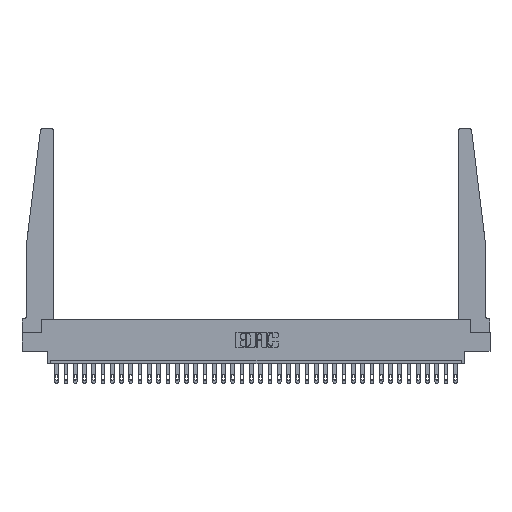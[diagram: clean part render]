
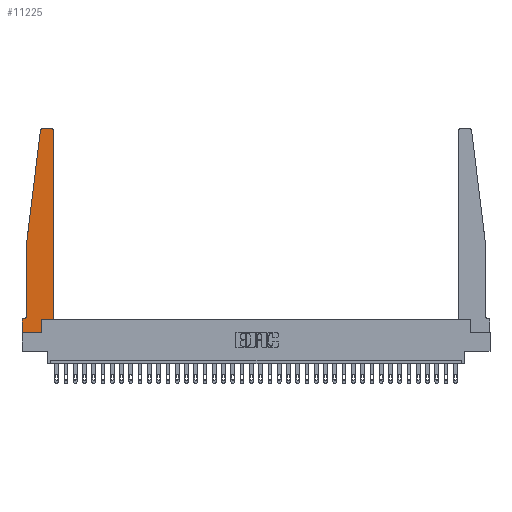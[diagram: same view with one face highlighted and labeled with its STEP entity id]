
A CAD part, top view. The second image highlights one B-rep face of the part: STEP entity #11225.
In plain terms, the highlighted planar face has unit normal (0, 0, 1).
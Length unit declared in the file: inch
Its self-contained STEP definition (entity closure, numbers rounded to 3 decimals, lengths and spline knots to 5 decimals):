
#347 = DIRECTION ( 'NONE',  ( 0., 1., 0. ) ) ;
#488 = DIRECTION ( 'NONE',  ( -1., 0., 0. ) ) ;
#572 = AXIS2_PLACEMENT_3D ( 'NONE', #25307, #10434, #15480 ) ;
#701 = VECTOR ( 'NONE', #6598, 39.37008 ) ;
#828 = VERTEX_POINT ( 'NONE', #2371 ) ;
#1574 = VERTEX_POINT ( 'NONE', #17901 ) ;
#1800 = CARTESIAN_POINT ( 'NONE',  ( 0., 0.1875, 0.37 ) ) ;
#2212 = EDGE_CURVE ( 'NONE', #27032, #22872, #29316, .T. ) ;
#2371 = CARTESIAN_POINT ( 'NONE',  ( 0.2605, 0., 0.37 ) ) ;
#2411 = PLANE ( 'NONE',  #4072 ) ;
#2854 = CIRCLE ( 'NONE', #22678, 0.03 ) ;
#3154 = LINE ( 'NONE', #15860, #17716 ) ;
#3325 = CARTESIAN_POINT ( 'NONE',  ( 0.015, 0.1875, 0.37 ) ) ;
#3471 = DIRECTION ( 'NONE',  ( 0., 1., 0. ) ) ;
#3914 = LINE ( 'NONE', #14338, #20668 ) ;
#4048 = DIRECTION ( 'NONE',  ( -1., 0., 0. ) ) ;
#4072 = AXIS2_PLACEMENT_3D ( 'NONE', #12355, #19717, #9597 ) ;
#4743 = CIRCLE ( 'NONE', #572, 0.03 ) ;
#4843 = CARTESIAN_POINT ( 'NONE',  ( 0.395, 2.75, 0.37 ) ) ;
#5253 = LINE ( 'NONE', #12909, #25466 ) ;
#5571 = CARTESIAN_POINT ( 'NONE',  ( 0.24675, 2.72367, 0.37 ) ) ;
#6073 = DIRECTION ( 'NONE',  ( -1., 0., 0. ) ) ;
#6445 = LINE ( 'NONE', #13642, #701 ) ;
#6598 = DIRECTION ( 'NONE',  ( -0.122, -0.992, 0. ) ) ;
#8385 = EDGE_LOOP ( 'NONE', ( #17911, #14973, #13995, #15410, #26064, #28689, #10773, #22045, #10524, #8840, #12205, #8422 ) ) ;
#8422 = ORIENTED_EDGE ( 'NONE', *, *, #14802, .T. ) ;
#8512 = LINE ( 'NONE', #26330, #14258 ) ;
#8748 = CARTESIAN_POINT ( 'NONE',  ( 0.2605, 0.18, 0.37 ) ) ;
#8840 = ORIENTED_EDGE ( 'NONE', *, *, #22077, .T. ) ;
#9363 = DIRECTION ( 'NONE',  ( 0., -1., 0. ) ) ;
#9597 = DIRECTION ( 'NONE',  ( 1., 0., 0. ) ) ;
#10434 = DIRECTION ( 'NONE',  ( 0., 0., 1. ) ) ;
#10437 = VERTEX_POINT ( 'NONE', #5571 ) ;
#10523 = EDGE_CURVE ( 'NONE', #18206, #24643, #25839, .T. ) ;
#10524 = ORIENTED_EDGE ( 'NONE', *, *, #16268, .T. ) ;
#10773 = ORIENTED_EDGE ( 'NONE', *, *, #30632, .T. ) ;
#11225 = ADVANCED_FACE ( 'NONE', ( #26758 ), #2411, .T. ) ;
#12205 = ORIENTED_EDGE ( 'NONE', *, *, #27524, .T. ) ;
#12355 = CARTESIAN_POINT ( 'NONE',  ( 0., 0.1875, 0.37 ) ) ;
#12909 = CARTESIAN_POINT ( 'NONE',  ( 0.425, 0.18, 0.37 ) ) ;
#13642 = CARTESIAN_POINT ( 'NONE',  ( 0.065, 1.25, 0.37 ) ) ;
#13995 = ORIENTED_EDGE ( 'NONE', *, *, #20664, .T. ) ;
#14258 = VECTOR ( 'NONE', #23366, 39.37008 ) ;
#14338 = CARTESIAN_POINT ( 'NONE',  ( 0., 0., 0.37 ) ) ;
#14802 = EDGE_CURVE ( 'NONE', #30425, #18206, #4743, .T. ) ;
#14973 = ORIENTED_EDGE ( 'NONE', *, *, #23504, .T. ) ;
#15410 = ORIENTED_EDGE ( 'NONE', *, *, #2212, .T. ) ;
#15480 = DIRECTION ( 'NONE',  ( 1., 0., 0. ) ) ;
#15860 = CARTESIAN_POINT ( 'NONE',  ( 0.2605, 0.18, 0.37 ) ) ;
#16268 = EDGE_CURVE ( 'NONE', #828, #25542, #3154, .T. ) ;
#16283 = CARTESIAN_POINT ( 'NONE',  ( 0.065, 0.1875, 0.37 ) ) ;
#17563 = CARTESIAN_POINT ( 'NONE',  ( 0., 0., 0.37 ) ) ;
#17716 = VECTOR ( 'NONE', #3471, 39.37008 ) ;
#17777 = CARTESIAN_POINT ( 'NONE',  ( 0.065, 0.2375, 0.37 ) ) ;
#17822 = CARTESIAN_POINT ( 'NONE',  ( 0.25, 2.75, 0.37 ) ) ;
#17901 = CARTESIAN_POINT ( 'NONE',  ( 0.425, 0.18, 0.37 ) ) ;
#17911 = ORIENTED_EDGE ( 'NONE', *, *, #10523, .T. ) ;
#18206 = VERTEX_POINT ( 'NONE', #4843 ) ;
#18893 = LINE ( 'NONE', #16283, #21741 ) ;
#19717 = DIRECTION ( 'NONE',  ( 0., 0., 1. ) ) ;
#20386 = EDGE_CURVE ( 'NONE', #23392, #828, #8512, .T. ) ;
#20664 = EDGE_CURVE ( 'NONE', #10437, #27032, #6445, .T. ) ;
#20668 = VECTOR ( 'NONE', #26150, 39.37008 ) ;
#21295 = CARTESIAN_POINT ( 'NONE',  ( 0.065, 1.25, 0.37 ) ) ;
#21338 = CARTESIAN_POINT ( 'NONE',  ( 0.015, 0.2375, 0.37 ) ) ;
#21658 = AXIS2_PLACEMENT_3D ( 'NONE', #21338, #25479, #488 ) ;
#21741 = VECTOR ( 'NONE', #4048, 39.37008 ) ;
#22045 = ORIENTED_EDGE ( 'NONE', *, *, #20386, .T. ) ;
#22047 = VERTEX_POINT ( 'NONE', #3325 ) ;
#22077 = EDGE_CURVE ( 'NONE', #25542, #1574, #22753, .T. ) ;
#22678 = AXIS2_PLACEMENT_3D ( 'NONE', #29342, #23770, #26878 ) ;
#22753 = LINE ( 'NONE', #25054, #24685 ) ;
#22872 = VERTEX_POINT ( 'NONE', #17777 ) ;
#23071 = DIRECTION ( 'NONE',  ( 1., 0., 0. ) ) ;
#23366 = DIRECTION ( 'NONE',  ( 1., 0., 0. ) ) ;
#23392 = VERTEX_POINT ( 'NONE', #17563 ) ;
#23504 = EDGE_CURVE ( 'NONE', #24643, #10437, #2854, .T. ) ;
#23770 = DIRECTION ( 'NONE',  ( 0., 0., 1. ) ) ;
#23916 = VERTEX_POINT ( 'NONE', #1800 ) ;
#24643 = VERTEX_POINT ( 'NONE', #26155 ) ;
#24685 = VECTOR ( 'NONE', #23071, 39.37008 ) ;
#25054 = CARTESIAN_POINT ( 'NONE',  ( 0.425, 0.18, 0.37 ) ) ;
#25307 = CARTESIAN_POINT ( 'NONE',  ( 0.395, 2.72, 0.37 ) ) ;
#25331 = CIRCLE ( 'NONE', #21658, 0.05 ) ;
#25466 = VECTOR ( 'NONE', #347, 39.37008 ) ;
#25479 = DIRECTION ( 'NONE',  ( 0., 0., -1. ) ) ;
#25542 = VERTEX_POINT ( 'NONE', #8748 ) ;
#25839 = LINE ( 'NONE', #17822, #28061 ) ;
#26064 = ORIENTED_EDGE ( 'NONE', *, *, #29300, .T. ) ;
#26150 = DIRECTION ( 'NONE',  ( 0., -1., 0. ) ) ;
#26155 = CARTESIAN_POINT ( 'NONE',  ( 0.27653, 2.75, 0.37 ) ) ;
#26330 = CARTESIAN_POINT ( 'NONE',  ( 0., 0., 0.37 ) ) ;
#26423 = EDGE_CURVE ( 'NONE', #22047, #23916, #18893, .T. ) ;
#26758 = FACE_OUTER_BOUND ( 'NONE', #8385, .T. ) ;
#26762 = VECTOR ( 'NONE', #9363, 39.37008 ) ;
#26878 = DIRECTION ( 'NONE',  ( 1., 0., 0. ) ) ;
#27032 = VERTEX_POINT ( 'NONE', #30148 ) ;
#27524 = EDGE_CURVE ( 'NONE', #1574, #30425, #5253, .T. ) ;
#27948 = CARTESIAN_POINT ( 'NONE',  ( 0.425, 2.72, 0.37 ) ) ;
#28061 = VECTOR ( 'NONE', #6073, 39.37008 ) ;
#28689 = ORIENTED_EDGE ( 'NONE', *, *, #26423, .T. ) ;
#29300 = EDGE_CURVE ( 'NONE', #22872, #22047, #25331, .T. ) ;
#29316 = LINE ( 'NONE', #21295, #26762 ) ;
#29342 = CARTESIAN_POINT ( 'NONE',  ( 0.27653, 2.72, 0.37 ) ) ;
#30148 = CARTESIAN_POINT ( 'NONE',  ( 0.065, 1.25, 0.37 ) ) ;
#30425 = VERTEX_POINT ( 'NONE', #27948 ) ;
#30632 = EDGE_CURVE ( 'NONE', #23916, #23392, #3914, .T. ) ;
